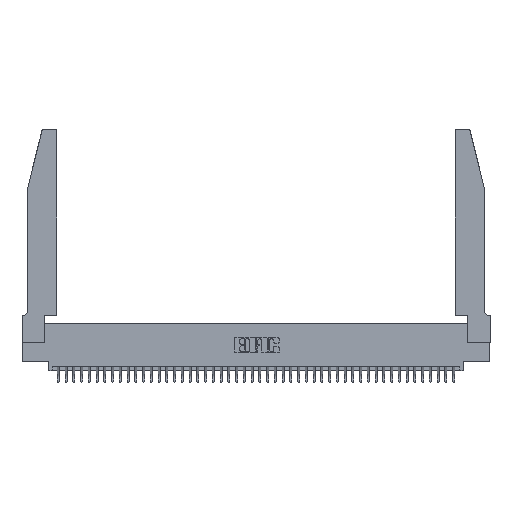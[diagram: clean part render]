
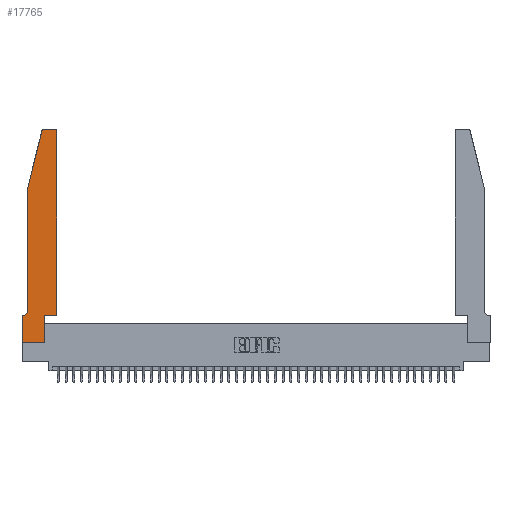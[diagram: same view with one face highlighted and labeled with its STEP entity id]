
A CAD part, top view. The second image highlights one B-rep face of the part: STEP entity #17765.
In plain terms, the highlighted planar face has unit normal (0, 0, 1).
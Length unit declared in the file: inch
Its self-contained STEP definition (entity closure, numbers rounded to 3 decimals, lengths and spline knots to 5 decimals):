
#116 = CARTESIAN_POINT ( 'NONE',  ( 0.0055, 0.35, 0.37 ) ) ;
#164 = DIRECTION ( 'NONE',  ( 1., 0., 0. ) ) ;
#455 = ORIENTED_EDGE ( 'NONE', *, *, #28303, .T. ) ;
#1034 = CARTESIAN_POINT ( 'NONE',  ( 0.0755, 0.35, 0.37 ) ) ;
#1053 = ORIENTED_EDGE ( 'NONE', *, *, #19403, .T. ) ;
#1583 = EDGE_CURVE ( 'NONE', #9643, #20237, #14915, .T. ) ;
#2160 = ORIENTED_EDGE ( 'NONE', *, *, #1583, .T. ) ;
#2397 = CARTESIAN_POINT ( 'NONE',  ( 0.284, 2.72, 0.37 ) ) ;
#3669 = CARTESIAN_POINT ( 'NONE',  ( 0.4505, 0.35, 0.37 ) ) ;
#4812 = CARTESIAN_POINT ( 'NONE',  ( 0.2865, 0., 0.37 ) ) ;
#5567 = CIRCLE ( 'NONE', #27389, 0.07 ) ;
#5965 = DIRECTION ( 'NONE',  ( 1., 0., 0. ) ) ;
#6528 = CIRCLE ( 'NONE', #9542, 0.03 ) ;
#6610 = CARTESIAN_POINT ( 'NONE',  ( 0.0055, 0.42, 0.37 ) ) ;
#6650 = EDGE_CURVE ( 'NONE', #9445, #42488, #38070, .T. ) ;
#7215 = DIRECTION ( 'NONE',  ( 0., 1., 0. ) ) ;
#7853 = CARTESIAN_POINT ( 'NONE',  ( 0.4505, 0.35, 0.37 ) ) ;
#9024 = FACE_OUTER_BOUND ( 'NONE', #27343, .T. ) ;
#9445 = VERTEX_POINT ( 'NONE', #116 ) ;
#9542 = AXIS2_PLACEMENT_3D ( 'NONE', #11438, #35316, #14882 ) ;
#9643 = VERTEX_POINT ( 'NONE', #4812 ) ;
#9927 = CARTESIAN_POINT ( 'NONE',  ( 0.2865, 0.35, 0.37 ) ) ;
#10140 = DIRECTION ( 'NONE',  ( -1., 0., 0. ) ) ;
#11438 = CARTESIAN_POINT ( 'NONE',  ( 0.4205, 2.72, 0.37 ) ) ;
#11927 = VECTOR ( 'NONE', #25299, 39.37008 ) ;
#12427 = CARTESIAN_POINT ( 'NONE',  ( 0.0755, 2., 0.37 ) ) ;
#12622 = VERTEX_POINT ( 'NONE', #28707 ) ;
#13195 = LINE ( 'NONE', #18278, #39320 ) ;
#13878 = CARTESIAN_POINT ( 'NONE',  ( 0., 0.35, 0.37 ) ) ;
#14032 = LINE ( 'NONE', #23830, #31101 ) ;
#14169 = CARTESIAN_POINT ( 'NONE',  ( 0., 0.35, 0.37 ) ) ;
#14693 = DIRECTION ( 'NONE',  ( 0., -1., 0. ) ) ;
#14882 = DIRECTION ( 'NONE',  ( 1., 0., 0. ) ) ;
#14915 = LINE ( 'NONE', #9927, #31986 ) ;
#15467 = CARTESIAN_POINT ( 'NONE',  ( 0.0755, 2., 0.37 ) ) ;
#15538 = CARTESIAN_POINT ( 'NONE',  ( 0.25487, 2.72718, 0.37 ) ) ;
#15819 = ORIENTED_EDGE ( 'NONE', *, *, #32026, .T. ) ;
#15861 = DIRECTION ( 'NONE',  ( -0.239, -0.971, 0. ) ) ;
#15905 = CARTESIAN_POINT ( 'NONE',  ( 0.4505, 0.35, 0.37 ) ) ;
#17094 = VECTOR ( 'NONE', #41941, 39.37008 ) ;
#17765 = ADVANCED_FACE ( 'NONE', ( #9024 ), #41444, .T. ) ;
#18164 = LINE ( 'NONE', #7853, #17094 ) ;
#18175 = VECTOR ( 'NONE', #43717, 39.37008 ) ;
#18278 = CARTESIAN_POINT ( 'NONE',  ( 0.0755, 2., 0.37 ) ) ;
#19100 = VERTEX_POINT ( 'NONE', #36906 ) ;
#19225 = LINE ( 'NONE', #23306, #18175 ) ;
#19403 = EDGE_CURVE ( 'NONE', #42488, #23065, #42026, .T. ) ;
#19587 = ORIENTED_EDGE ( 'NONE', *, *, #36321, .T. ) ;
#19746 = LINE ( 'NONE', #3669, #36806 ) ;
#20237 = VERTEX_POINT ( 'NONE', #35805 ) ;
#20796 = EDGE_CURVE ( 'NONE', #12622, #27141, #6528, .T. ) ;
#21040 = DIRECTION ( 'NONE',  ( 0., 0., 1. ) ) ;
#21695 = DIRECTION ( 'NONE',  ( 0., -1., 0. ) ) ;
#22510 = VERTEX_POINT ( 'NONE', #25751 ) ;
#22784 = ORIENTED_EDGE ( 'NONE', *, *, #35705, .T. ) ;
#23062 = EDGE_CURVE ( 'NONE', #22510, #9445, #5567, .T. ) ;
#23065 = VERTEX_POINT ( 'NONE', #44164 ) ;
#23306 = CARTESIAN_POINT ( 'NONE',  ( 0., 0., 0.37 ) ) ;
#23454 = VERTEX_POINT ( 'NONE', #15538 ) ;
#23830 = CARTESIAN_POINT ( 'NONE',  ( 0.2605, 2.75, 0.37 ) ) ;
#25299 = DIRECTION ( 'NONE',  ( -1., 0., 0. ) ) ;
#25751 = CARTESIAN_POINT ( 'NONE',  ( 0.0755, 0.42, 0.37 ) ) ;
#26568 = DIRECTION ( 'NONE',  ( 0., 0., 1. ) ) ;
#27024 = ORIENTED_EDGE ( 'NONE', *, *, #43610, .T. ) ;
#27141 = VERTEX_POINT ( 'NONE', #32182 ) ;
#27261 = DIRECTION ( 'NONE',  ( -1., 0., 0. ) ) ;
#27343 = EDGE_LOOP ( 'NONE', ( #15819, #27024, #455, #30237, #31325, #34543, #1053, #19587, #2160, #22784, #31888, #43051 ) ) ;
#27389 = AXIS2_PLACEMENT_3D ( 'NONE', #6610, #30627, #10140 ) ;
#28303 = EDGE_CURVE ( 'NONE', #23454, #32447, #29827, .T. ) ;
#28707 = CARTESIAN_POINT ( 'NONE',  ( 0.4505, 2.72, 0.37 ) ) ;
#29565 = VERTEX_POINT ( 'NONE', #15905 ) ;
#29827 = LINE ( 'NONE', #12427, #36743 ) ;
#30132 = AXIS2_PLACEMENT_3D ( 'NONE', #14169, #21040, #164 ) ;
#30237 = ORIENTED_EDGE ( 'NONE', *, *, #38020, .T. ) ;
#30627 = DIRECTION ( 'NONE',  ( 0., 0., -1. ) ) ;
#31101 = VECTOR ( 'NONE', #27261, 39.37008 ) ;
#31325 = ORIENTED_EDGE ( 'NONE', *, *, #23062, .T. ) ;
#31696 = CARTESIAN_POINT ( 'NONE',  ( 0., 0., 0.37 ) ) ;
#31888 = ORIENTED_EDGE ( 'NONE', *, *, #36515, .T. ) ;
#31901 = VECTOR ( 'NONE', #14693, 39.37008 ) ;
#31986 = VECTOR ( 'NONE', #40692, 39.37008 ) ;
#32026 = EDGE_CURVE ( 'NONE', #27141, #19100, #14032, .T. ) ;
#32182 = CARTESIAN_POINT ( 'NONE',  ( 0.4205, 2.75, 0.37 ) ) ;
#32447 = VERTEX_POINT ( 'NONE', #15467 ) ;
#34543 = ORIENTED_EDGE ( 'NONE', *, *, #6650, .T. ) ;
#35316 = DIRECTION ( 'NONE',  ( 0., 0., 1. ) ) ;
#35705 = EDGE_CURVE ( 'NONE', #20237, #29565, #18164, .T. ) ;
#35805 = CARTESIAN_POINT ( 'NONE',  ( 0.2865, 0.35, 0.37 ) ) ;
#36321 = EDGE_CURVE ( 'NONE', #23065, #9643, #19225, .T. ) ;
#36515 = EDGE_CURVE ( 'NONE', #29565, #12622, #19746, .T. ) ;
#36743 = VECTOR ( 'NONE', #15861, 39.37008 ) ;
#36806 = VECTOR ( 'NONE', #7215, 39.37008 ) ;
#36906 = CARTESIAN_POINT ( 'NONE',  ( 0.284, 2.75, 0.37 ) ) ;
#38020 = EDGE_CURVE ( 'NONE', #32447, #22510, #13195, .T. ) ;
#38070 = LINE ( 'NONE', #1034, #11927 ) ;
#39320 = VECTOR ( 'NONE', #21695, 39.37008 ) ;
#40692 = DIRECTION ( 'NONE',  ( 0., 1., 0. ) ) ;
#41444 = PLANE ( 'NONE',  #30132 ) ;
#41941 = DIRECTION ( 'NONE',  ( 1., 0., 0. ) ) ;
#42026 = LINE ( 'NONE', #31696, #31901 ) ;
#42488 = VERTEX_POINT ( 'NONE', #13878 ) ;
#43051 = ORIENTED_EDGE ( 'NONE', *, *, #20796, .T. ) ;
#43308 = AXIS2_PLACEMENT_3D ( 'NONE', #2397, #26568, #5965 ) ;
#43610 = EDGE_CURVE ( 'NONE', #19100, #23454, #44143, .T. ) ;
#43717 = DIRECTION ( 'NONE',  ( 1., 0., 0. ) ) ;
#44143 = CIRCLE ( 'NONE', #43308, 0.03 ) ;
#44164 = CARTESIAN_POINT ( 'NONE',  ( 0., 0., 0.37 ) ) ;
